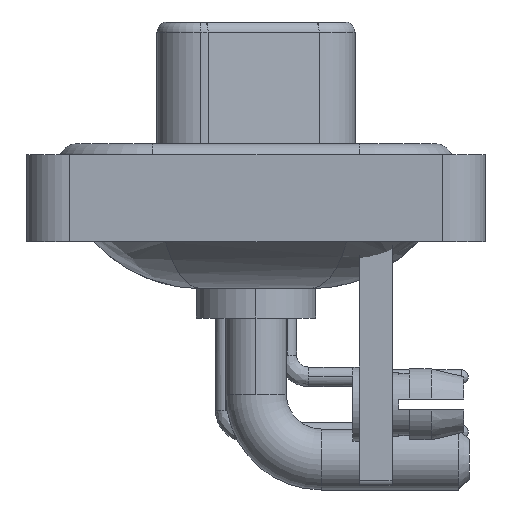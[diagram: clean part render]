
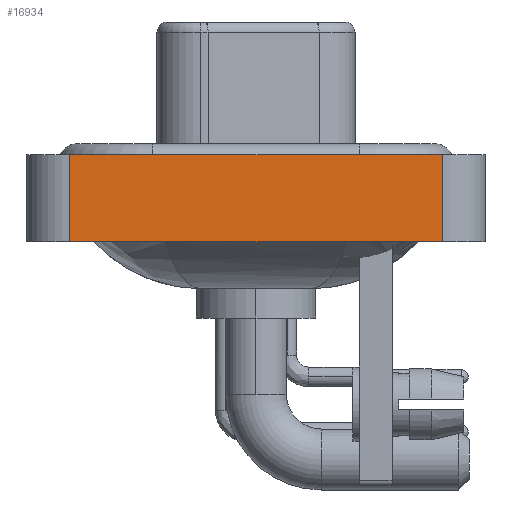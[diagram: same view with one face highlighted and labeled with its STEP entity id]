
A CAD part, left-side view. The second image highlights one B-rep face of the part: STEP entity #16934.
In plain terms, the highlighted planar face has unit normal (-1, 0, 0).
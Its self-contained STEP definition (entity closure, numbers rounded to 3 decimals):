
#69 = DIRECTION ( 'NONE',  ( 0., 0., 1. ) ) ;
#189 = ORIENTED_EDGE ( 'NONE', *, *, #19667, .T. ) ;
#4027 = VERTEX_POINT ( 'NONE', #22909 ) ;
#4116 = CARTESIAN_POINT ( 'NONE',  ( -7.35, 8.55, -3.6 ) ) ;
#5344 = CARTESIAN_POINT ( 'NONE',  ( -7.35, -8.55, -3.6 ) ) ;
#5717 = VECTOR ( 'NONE', #16487, 1000. ) ;
#5737 = ORIENTED_EDGE ( 'NONE', *, *, #25790, .T. ) ;
#6035 = EDGE_LOOP ( 'NONE', ( #5737, #21246, #15246, #189 ) ) ;
#6546 = DIRECTION ( 'NONE',  ( 0., 0., 1. ) ) ;
#7811 = VECTOR ( 'NONE', #24769, 1000. ) ;
#7883 = PLANE ( 'NONE',  #25209 ) ;
#10648 = VERTEX_POINT ( 'NONE', #19358 ) ;
#10992 = VECTOR ( 'NONE', #69, 1000. ) ;
#11543 = EDGE_CURVE ( 'NONE', #10648, #4027, #23881, .T. ) ;
#12147 = VERTEX_POINT ( 'NONE', #24552 ) ;
#13530 = LINE ( 'NONE', #15702, #7811 ) ;
#14260 = FACE_OUTER_BOUND ( 'NONE', #6035, .T. ) ;
#14398 = DIRECTION ( 'NONE',  ( -1., 0., 0. ) ) ;
#15246 = ORIENTED_EDGE ( 'NONE', *, *, #11543, .F. ) ;
#15466 = VECTOR ( 'NONE', #6546, 1000. ) ;
#15702 = CARTESIAN_POINT ( 'NONE',  ( -7.35, -8.55, 0.4 ) ) ;
#16487 = DIRECTION ( 'NONE',  ( 0., -1., 0. ) ) ;
#16934 = ADVANCED_FACE ( 'NONE', ( #14260 ), #7883, .T. ) ;
#18056 = LINE ( 'NONE', #5344, #5717 ) ;
#19358 = CARTESIAN_POINT ( 'NONE',  ( -7.35, 8.55, -3.6 ) ) ;
#19667 = EDGE_CURVE ( 'NONE', #10648, #12147, #18056, .T. ) ;
#19924 = CARTESIAN_POINT ( 'NONE',  ( -7.35, -8.55, -3.6 ) ) ;
#20584 = CARTESIAN_POINT ( 'NONE',  ( -7.35, -8.55, -3.6 ) ) ;
#21246 = ORIENTED_EDGE ( 'NONE', *, *, #26913, .F. ) ;
#22909 = CARTESIAN_POINT ( 'NONE',  ( -7.35, 8.55, 0.4 ) ) ;
#23665 = VERTEX_POINT ( 'NONE', #23933 ) ;
#23881 = LINE ( 'NONE', #4116, #15466 ) ;
#23933 = CARTESIAN_POINT ( 'NONE',  ( -7.35, -8.55, 0.4 ) ) ;
#24552 = CARTESIAN_POINT ( 'NONE',  ( -7.35, -8.55, -3.6 ) ) ;
#24769 = DIRECTION ( 'NONE',  ( 0., -1., 0. ) ) ;
#25199 = DIRECTION ( 'NONE',  ( 0., 0., 1. ) ) ;
#25209 = AXIS2_PLACEMENT_3D ( 'NONE', #20584, #14398, #25199 ) ;
#25790 = EDGE_CURVE ( 'NONE', #12147, #23665, #26140, .T. ) ;
#26140 = LINE ( 'NONE', #19924, #10992 ) ;
#26913 = EDGE_CURVE ( 'NONE', #4027, #23665, #13530, .T. ) ;
